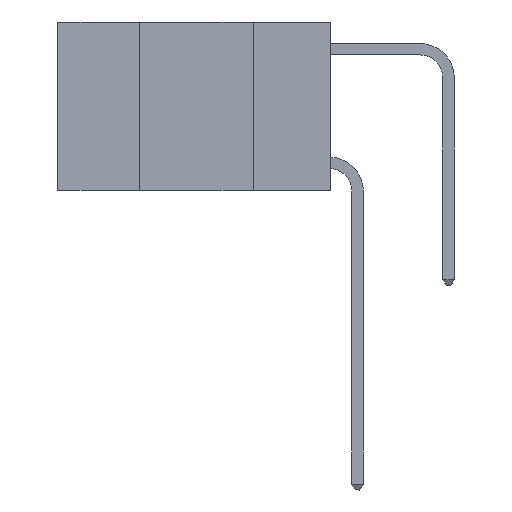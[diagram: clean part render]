
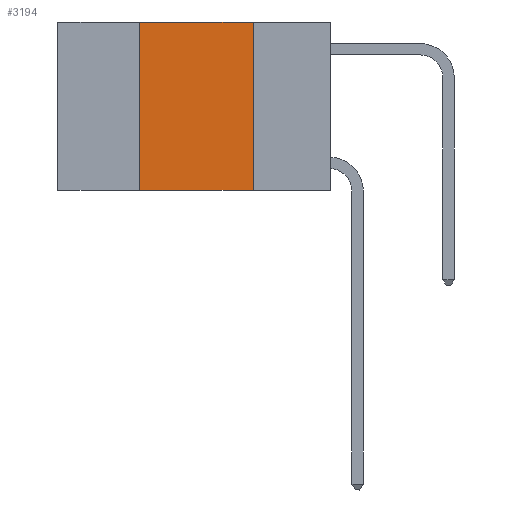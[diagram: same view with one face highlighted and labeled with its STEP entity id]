
A CAD part, left-side view. The second image highlights one B-rep face of the part: STEP entity #3194.
In plain terms, the highlighted planar face has unit normal (-1, 0, 0).
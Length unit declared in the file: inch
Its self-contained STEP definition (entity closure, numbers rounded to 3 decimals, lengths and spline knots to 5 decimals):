
#1 = VERTEX_POINT ( 'NONE', #7313 ) ;
#151 = EDGE_CURVE ( 'NONE', #10657, #1, #961, .T. ) ;
#179 = ORIENTED_EDGE ( 'NONE', *, *, #151, .F. ) ;
#520 = CARTESIAN_POINT ( 'NONE',  ( 0., 0.6, -0.37 ) ) ;
#961 = LINE ( 'NONE', #6820, #4674 ) ;
#1343 = CARTESIAN_POINT ( 'NONE',  ( 0., 0.42, 0. ) ) ;
#1444 = LINE ( 'NONE', #3614, #10805 ) ;
#1695 = VECTOR ( 'NONE', #11392, 39.37008 ) ;
#1785 = VERTEX_POINT ( 'NONE', #2330 ) ;
#2330 = CARTESIAN_POINT ( 'NONE',  ( 0., 0.17, -0.37 ) ) ;
#2367 = ORIENTED_EDGE ( 'NONE', *, *, #6910, .F. ) ;
#3038 = EDGE_CURVE ( 'NONE', #7574, #10657, #4755, .T. ) ;
#3194 = ADVANCED_FACE ( 'NONE', ( #8179 ), #7072, .F. ) ;
#3477 = DIRECTION ( 'NONE',  ( 0., 0., -1. ) ) ;
#3614 = CARTESIAN_POINT ( 'NONE',  ( 0., 0.17, 0. ) ) ;
#4088 = ORIENTED_EDGE ( 'NONE', *, *, #3038, .F. ) ;
#4588 = CARTESIAN_POINT ( 'NONE',  ( 0., 0.42, -0.37 ) ) ;
#4674 = VECTOR ( 'NONE', #6288, 39.37008 ) ;
#4755 = LINE ( 'NONE', #1343, #9271 ) ;
#5352 = CARTESIAN_POINT ( 'NONE',  ( 0., 0.6, 0. ) ) ;
#5452 = DIRECTION ( 'NONE',  ( 0., 0., -1. ) ) ;
#5611 = DIRECTION ( 'NONE',  ( 0., 0., 1. ) ) ;
#5792 = EDGE_LOOP ( 'NONE', ( #2367, #179, #4088, #10482 ) ) ;
#6288 = DIRECTION ( 'NONE',  ( 0., -1., 0. ) ) ;
#6591 = CARTESIAN_POINT ( 'NONE',  ( 0., 0.42, 0. ) ) ;
#6820 = CARTESIAN_POINT ( 'NONE',  ( 0., 0.6, 0. ) ) ;
#6861 = LINE ( 'NONE', #520, #1695 ) ;
#6910 = EDGE_CURVE ( 'NONE', #1, #1785, #1444, .T. ) ;
#7072 = PLANE ( 'NONE',  #11193 ) ;
#7313 = CARTESIAN_POINT ( 'NONE',  ( 0., 0.17, 0. ) ) ;
#7574 = VERTEX_POINT ( 'NONE', #4588 ) ;
#8179 = FACE_OUTER_BOUND ( 'NONE', #5792, .T. ) ;
#9114 = EDGE_CURVE ( 'NONE', #7574, #1785, #6861, .T. ) ;
#9271 = VECTOR ( 'NONE', #5611, 39.37008 ) ;
#9646 = DIRECTION ( 'NONE',  ( 1., 0., 0. ) ) ;
#10482 = ORIENTED_EDGE ( 'NONE', *, *, #9114, .T. ) ;
#10657 = VERTEX_POINT ( 'NONE', #6591 ) ;
#10805 = VECTOR ( 'NONE', #5452, 39.37008 ) ;
#11193 = AXIS2_PLACEMENT_3D ( 'NONE', #5352, #9646, #3477 ) ;
#11392 = DIRECTION ( 'NONE',  ( 0., -1., 0. ) ) ;
